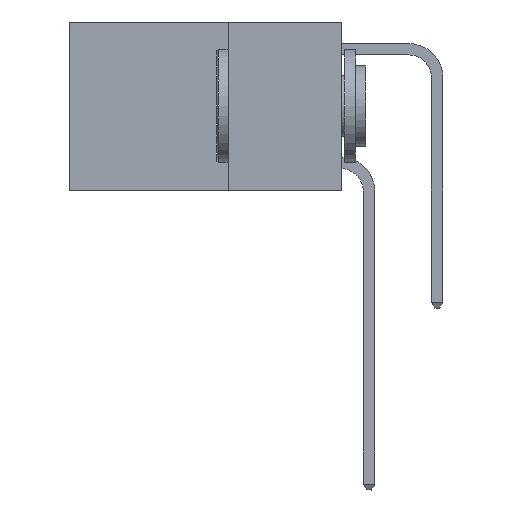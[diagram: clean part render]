
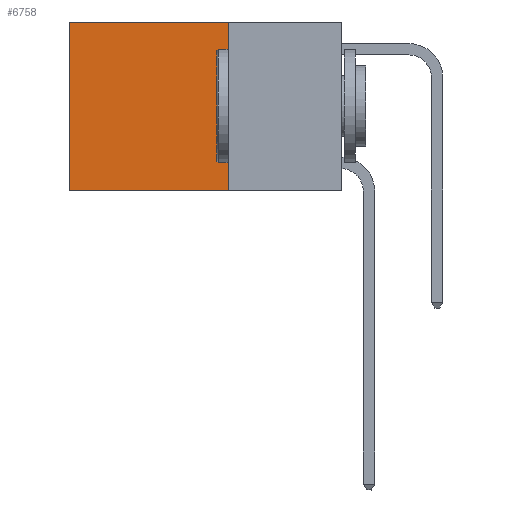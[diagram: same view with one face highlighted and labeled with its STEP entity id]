
A CAD part, left-side view. The second image highlights one B-rep face of the part: STEP entity #6758.
In plain terms, the highlighted planar face has unit normal (-1, 0, 0).
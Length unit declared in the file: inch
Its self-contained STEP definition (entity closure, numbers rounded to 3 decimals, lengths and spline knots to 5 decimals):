
#2587 = ORIENTED_EDGE ( 'NONE', *, *, #13864, .T. ) ;
#3626 = VERTEX_POINT ( 'NONE', #12239 ) ;
#4693 = VERTEX_POINT ( 'NONE', #24636 ) ;
#5610 = CARTESIAN_POINT ( 'NONE',  ( 0.2625, 0.25, 0. ) ) ;
#5799 = ORIENTED_EDGE ( 'NONE', *, *, #26005, .F. ) ;
#5847 = EDGE_CURVE ( 'NONE', #4693, #10889, #26525, .T. ) ;
#6758 = ADVANCED_FACE ( 'NONE', ( #13907 ), #12001, .F. ) ;
#8684 = EDGE_CURVE ( 'NONE', #3626, #23415, #20789, .T. ) ;
#10889 = VERTEX_POINT ( 'NONE', #15175 ) ;
#11275 = DIRECTION ( 'NONE',  ( 0., 1., 0. ) ) ;
#12001 = PLANE ( 'NONE',  #12334 ) ;
#12239 = CARTESIAN_POINT ( 'NONE',  ( 0.2625, 0.6, 0. ) ) ;
#12334 = AXIS2_PLACEMENT_3D ( 'NONE', #32295, #22291, #20649 ) ;
#12528 = DIRECTION ( 'NONE',  ( 0., 0., -1. ) ) ;
#13864 = EDGE_CURVE ( 'NONE', #4693, #3626, #20977, .T. ) ;
#13907 = FACE_OUTER_BOUND ( 'NONE', #19243, .T. ) ;
#14276 = ORIENTED_EDGE ( 'NONE', *, *, #5847, .F. ) ;
#15175 = CARTESIAN_POINT ( 'NONE',  ( 0.2625, 0.25, -0.37 ) ) ;
#16875 = CARTESIAN_POINT ( 'NONE',  ( 0.2625, 0.25, 0. ) ) ;
#17731 = VECTOR ( 'NONE', #11275, 39.37008 ) ;
#19243 = EDGE_LOOP ( 'NONE', ( #26965, #5799, #14276, #2587 ) ) ;
#20028 = VECTOR ( 'NONE', #12528, 39.37008 ) ;
#20649 = DIRECTION ( 'NONE',  ( 0., 0., -1. ) ) ;
#20789 = LINE ( 'NONE', #22496, #20028 ) ;
#20977 = LINE ( 'NONE', #5610, #22574 ) ;
#22291 = DIRECTION ( 'NONE',  ( 1., 0., 0. ) ) ;
#22496 = CARTESIAN_POINT ( 'NONE',  ( 0.2625, 0.6, 0. ) ) ;
#22574 = VECTOR ( 'NONE', #28243, 39.37008 ) ;
#23415 = VERTEX_POINT ( 'NONE', #30146 ) ;
#23995 = CARTESIAN_POINT ( 'NONE',  ( 0.2625, 0.25, -0.37 ) ) ;
#24636 = CARTESIAN_POINT ( 'NONE',  ( 0.2625, 0.25, 0. ) ) ;
#26005 = EDGE_CURVE ( 'NONE', #10889, #23415, #29962, .T. ) ;
#26525 = LINE ( 'NONE', #16875, #30863 ) ;
#26965 = ORIENTED_EDGE ( 'NONE', *, *, #8684, .T. ) ;
#28243 = DIRECTION ( 'NONE',  ( 0., 1., 0. ) ) ;
#29099 = DIRECTION ( 'NONE',  ( 0., 0., -1. ) ) ;
#29962 = LINE ( 'NONE', #23995, #17731 ) ;
#30146 = CARTESIAN_POINT ( 'NONE',  ( 0.2625, 0.6, -0.37 ) ) ;
#30863 = VECTOR ( 'NONE', #29099, 39.37008 ) ;
#32295 = CARTESIAN_POINT ( 'NONE',  ( 0.2625, 0.25, 0. ) ) ;
